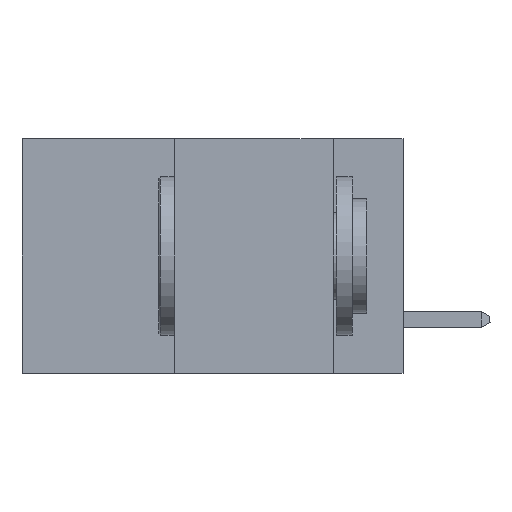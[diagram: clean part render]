
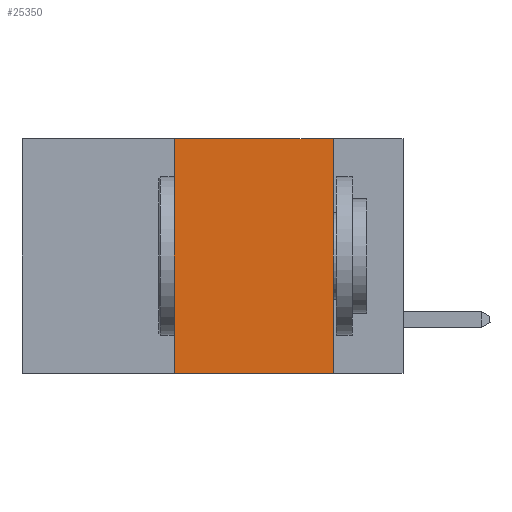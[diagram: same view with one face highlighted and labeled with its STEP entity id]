
A CAD part, left-side view. The second image highlights one B-rep face of the part: STEP entity #25350.
In plain terms, the highlighted planar face has unit normal (-1, 0, 0).
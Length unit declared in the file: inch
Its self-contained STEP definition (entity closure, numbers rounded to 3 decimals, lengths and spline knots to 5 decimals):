
#2430 = CARTESIAN_POINT ( 'NONE',  ( 0., 0.6, 0. ) ) ;
#3889 = CARTESIAN_POINT ( 'NONE',  ( 0., 0.11, 0. ) ) ;
#4321 = VECTOR ( 'NONE', #4572, 39.37008 ) ;
#4572 = DIRECTION ( 'NONE',  ( 0., 0., 1. ) ) ;
#4678 = CARTESIAN_POINT ( 'NONE',  ( 0., 0.6, 0. ) ) ;
#5994 = CARTESIAN_POINT ( 'NONE',  ( 0., 0.36, 0. ) ) ;
#6497 = CARTESIAN_POINT ( 'NONE',  ( 0., 0.11, -0.37 ) ) ;
#7579 = CARTESIAN_POINT ( 'NONE',  ( 0., 0.36, 0. ) ) ;
#7826 = DIRECTION ( 'NONE',  ( 0., 0., -1. ) ) ;
#10051 = DIRECTION ( 'NONE',  ( 0., 0., -1. ) ) ;
#13233 = EDGE_LOOP ( 'NONE', ( #29387, #34687, #24968, #21691 ) ) ;
#13779 = CARTESIAN_POINT ( 'NONE',  ( 0., 0.11, 0. ) ) ;
#13992 = VERTEX_POINT ( 'NONE', #6497 ) ;
#17567 = EDGE_CURVE ( 'NONE', #23981, #37028, #29774, .T. ) ;
#18325 = EDGE_CURVE ( 'NONE', #37028, #22233, #26997, .T. ) ;
#18903 = AXIS2_PLACEMENT_3D ( 'NONE', #4678, #26603, #7826 ) ;
#20536 = DIRECTION ( 'NONE',  ( 0., -1., 0. ) ) ;
#21075 = VECTOR ( 'NONE', #20536, 39.37008 ) ;
#21102 = VECTOR ( 'NONE', #39545, 39.37008 ) ;
#21691 = ORIENTED_EDGE ( 'NONE', *, *, #39899, .T. ) ;
#22233 = VERTEX_POINT ( 'NONE', #13779 ) ;
#22246 = FACE_OUTER_BOUND ( 'NONE', #13233, .T. ) ;
#23981 = VERTEX_POINT ( 'NONE', #31112 ) ;
#24968 = ORIENTED_EDGE ( 'NONE', *, *, #17567, .F. ) ;
#25350 = ADVANCED_FACE ( 'NONE', ( #22246 ), #35815, .F. ) ;
#26603 = DIRECTION ( 'NONE',  ( 1., 0., 0. ) ) ;
#26671 = LINE ( 'NONE', #3889, #32030 ) ;
#26997 = LINE ( 'NONE', #2430, #21102 ) ;
#27112 = CARTESIAN_POINT ( 'NONE',  ( 0., 0.6, -0.37 ) ) ;
#29387 = ORIENTED_EDGE ( 'NONE', *, *, #35121, .F. ) ;
#29774 = LINE ( 'NONE', #7579, #4321 ) ;
#31112 = CARTESIAN_POINT ( 'NONE',  ( 0., 0.36, -0.37 ) ) ;
#32030 = VECTOR ( 'NONE', #10051, 39.37008 ) ;
#34687 = ORIENTED_EDGE ( 'NONE', *, *, #18325, .F. ) ;
#35121 = EDGE_CURVE ( 'NONE', #22233, #13992, #26671, .T. ) ;
#35815 = PLANE ( 'NONE',  #18903 ) ;
#36651 = LINE ( 'NONE', #27112, #21075 ) ;
#37028 = VERTEX_POINT ( 'NONE', #5994 ) ;
#39545 = DIRECTION ( 'NONE',  ( 0., -1., 0. ) ) ;
#39899 = EDGE_CURVE ( 'NONE', #23981, #13992, #36651, .T. ) ;
